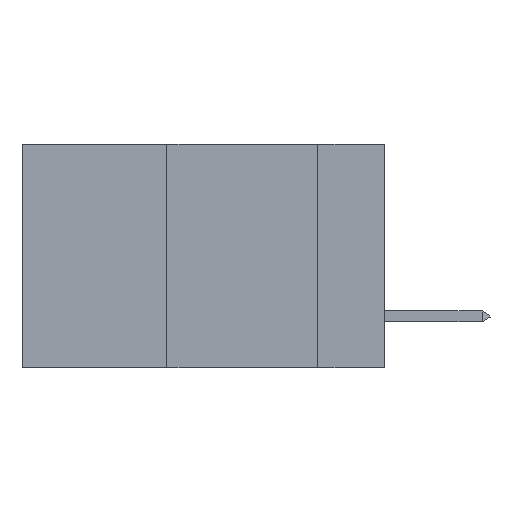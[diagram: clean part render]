
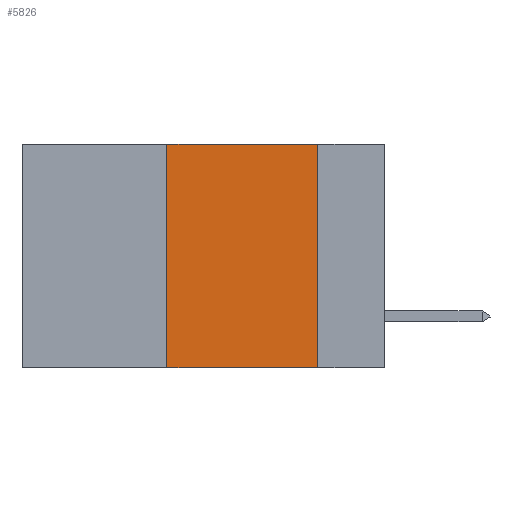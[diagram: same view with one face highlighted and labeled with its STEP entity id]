
A CAD part, left-side view. The second image highlights one B-rep face of the part: STEP entity #5826.
In plain terms, the highlighted planar face has unit normal (-1, 0, 0).
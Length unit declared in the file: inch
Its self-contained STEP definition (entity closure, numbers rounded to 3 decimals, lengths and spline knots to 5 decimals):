
#1243 = LINE ( 'NONE', #20508, #23749 ) ;
#2090 = CARTESIAN_POINT ( 'NONE',  ( 0., 0.6, 0. ) ) ;
#2305 = EDGE_CURVE ( 'NONE', #5382, #5267, #21363, .T. ) ;
#3080 = EDGE_CURVE ( 'NONE', #23040, #11679, #20197, .T. ) ;
#3172 = EDGE_LOOP ( 'NONE', ( #26213, #26149, #16692, #11226 ) ) ;
#3227 = PLANE ( 'NONE',  #8296 ) ;
#5267 = VERTEX_POINT ( 'NONE', #45644 ) ;
#5382 = VERTEX_POINT ( 'NONE', #19278 ) ;
#5826 = ADVANCED_FACE ( 'NONE', ( #31807 ), #3227, .F. ) ;
#8158 = LINE ( 'NONE', #2090, #45344 ) ;
#8296 = AXIS2_PLACEMENT_3D ( 'NONE', #16876, #10151, #31900 ) ;
#9005 = DIRECTION ( 'NONE',  ( 0., -1., 0. ) ) ;
#10151 = DIRECTION ( 'NONE',  ( 1., 0., 0. ) ) ;
#11226 = ORIENTED_EDGE ( 'NONE', *, *, #17896, .T. ) ;
#11679 = VERTEX_POINT ( 'NONE', #44022 ) ;
#12847 = DIRECTION ( 'NONE',  ( 0., 0., -1. ) ) ;
#16692 = ORIENTED_EDGE ( 'NONE', *, *, #2305, .F. ) ;
#16876 = CARTESIAN_POINT ( 'NONE',  ( 0., 0.6, 0. ) ) ;
#17896 = EDGE_CURVE ( 'NONE', #5382, #11679, #1243, .T. ) ;
#19278 = CARTESIAN_POINT ( 'NONE',  ( 0., 0.36, -0.37 ) ) ;
#20155 = CARTESIAN_POINT ( 'NONE',  ( 0., 0.11, 0. ) ) ;
#20197 = LINE ( 'NONE', #20155, #21871 ) ;
#20508 = CARTESIAN_POINT ( 'NONE',  ( 0., 0.6, -0.37 ) ) ;
#21363 = LINE ( 'NONE', #32210, #45116 ) ;
#21871 = VECTOR ( 'NONE', #12847, 39.37008 ) ;
#23040 = VERTEX_POINT ( 'NONE', #42636 ) ;
#23749 = VECTOR ( 'NONE', #27173, 39.37008 ) ;
#26149 = ORIENTED_EDGE ( 'NONE', *, *, #27921, .F. ) ;
#26213 = ORIENTED_EDGE ( 'NONE', *, *, #3080, .F. ) ;
#27173 = DIRECTION ( 'NONE',  ( 0., -1., 0. ) ) ;
#27921 = EDGE_CURVE ( 'NONE', #5267, #23040, #8158, .T. ) ;
#31807 = FACE_OUTER_BOUND ( 'NONE', #3172, .T. ) ;
#31900 = DIRECTION ( 'NONE',  ( 0., 0., -1. ) ) ;
#32210 = CARTESIAN_POINT ( 'NONE',  ( 0., 0.36, 0. ) ) ;
#32375 = DIRECTION ( 'NONE',  ( 0., 0., 1. ) ) ;
#42636 = CARTESIAN_POINT ( 'NONE',  ( 0., 0.11, 0. ) ) ;
#44022 = CARTESIAN_POINT ( 'NONE',  ( 0., 0.11, -0.37 ) ) ;
#45116 = VECTOR ( 'NONE', #32375, 39.37008 ) ;
#45344 = VECTOR ( 'NONE', #9005, 39.37008 ) ;
#45644 = CARTESIAN_POINT ( 'NONE',  ( 0., 0.36, 0. ) ) ;
